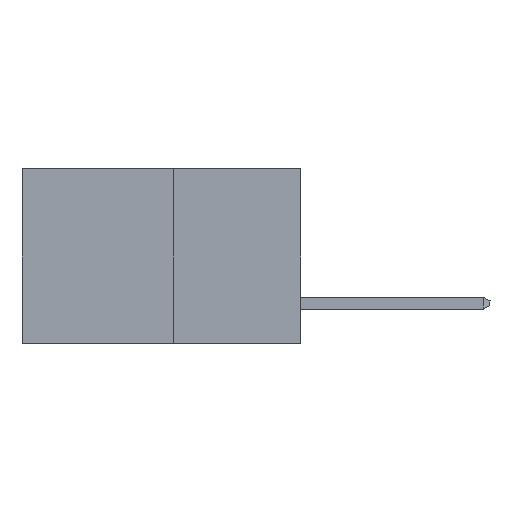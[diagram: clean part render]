
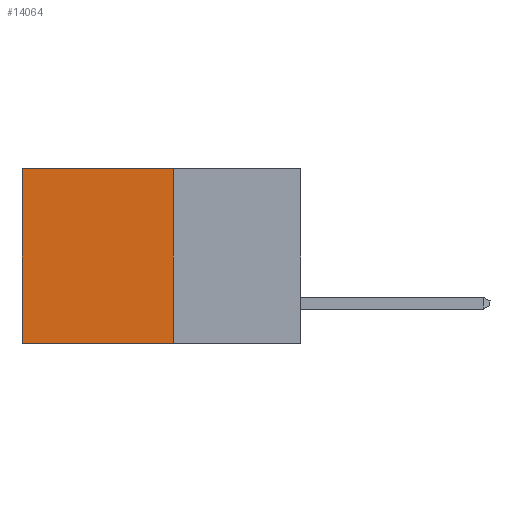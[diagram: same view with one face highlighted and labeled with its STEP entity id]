
A CAD part, left-side view. The second image highlights one B-rep face of the part: STEP entity #14064.
In plain terms, the highlighted planar face has unit normal (-1, 0, 0).
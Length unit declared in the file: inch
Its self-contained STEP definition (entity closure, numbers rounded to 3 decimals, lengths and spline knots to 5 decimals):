
#229 = ORIENTED_EDGE ( 'NONE', *, *, #17463, .F. ) ;
#1659 = VECTOR ( 'NONE', #18160, 39.37008 ) ;
#1755 = DIRECTION ( 'NONE',  ( 0., 1., 0. ) ) ;
#2452 = LINE ( 'NONE', #6009, #1659 ) ;
#3573 = DIRECTION ( 'NONE',  ( 1., 0., 0. ) ) ;
#4290 = LINE ( 'NONE', #23374, #28162 ) ;
#5019 = LINE ( 'NONE', #24667, #23344 ) ;
#5097 = CARTESIAN_POINT ( 'NONE',  ( 0.277, 0.59, 0. ) ) ;
#6009 = CARTESIAN_POINT ( 'NONE',  ( 0.277, 0.27, -0.37 ) ) ;
#6971 = VECTOR ( 'NONE', #15174, 39.37008 ) ;
#7074 = EDGE_CURVE ( 'NONE', #9662, #13632, #20479, .T. ) ;
#8551 = EDGE_LOOP ( 'NONE', ( #28780, #25128, #229, #24511 ) ) ;
#9662 = VERTEX_POINT ( 'NONE', #5097 ) ;
#10799 = PLANE ( 'NONE',  #11037 ) ;
#11037 = AXIS2_PLACEMENT_3D ( 'NONE', #24956, #3573, #20393 ) ;
#11593 = VERTEX_POINT ( 'NONE', #11959 ) ;
#11959 = CARTESIAN_POINT ( 'NONE',  ( 0.277, 0.27, -0.37 ) ) ;
#13632 = VERTEX_POINT ( 'NONE', #13895 ) ;
#13895 = CARTESIAN_POINT ( 'NONE',  ( 0.277, 0.59, -0.37 ) ) ;
#14064 = ADVANCED_FACE ( 'NONE', ( #22107 ), #10799, .F. ) ;
#15174 = DIRECTION ( 'NONE',  ( 0., 0., -1. ) ) ;
#17062 = EDGE_CURVE ( 'NONE', #23329, #9662, #4290, .T. ) ;
#17463 = EDGE_CURVE ( 'NONE', #23329, #11593, #5019, .T. ) ;
#18160 = DIRECTION ( 'NONE',  ( 0., 1., 0. ) ) ;
#20393 = DIRECTION ( 'NONE',  ( 0., 0., -1. ) ) ;
#20479 = LINE ( 'NONE', #24603, #6971 ) ;
#22107 = FACE_OUTER_BOUND ( 'NONE', #8551, .T. ) ;
#22429 = DIRECTION ( 'NONE',  ( 0., 0., -1. ) ) ;
#23329 = VERTEX_POINT ( 'NONE', #24039 ) ;
#23344 = VECTOR ( 'NONE', #22429, 39.37008 ) ;
#23374 = CARTESIAN_POINT ( 'NONE',  ( 0.277, 0.27, 0. ) ) ;
#24039 = CARTESIAN_POINT ( 'NONE',  ( 0.277, 0.27, 0. ) ) ;
#24511 = ORIENTED_EDGE ( 'NONE', *, *, #17062, .T. ) ;
#24603 = CARTESIAN_POINT ( 'NONE',  ( 0.277, 0.59, -0.37 ) ) ;
#24667 = CARTESIAN_POINT ( 'NONE',  ( 0.277, 0.27, -0.37 ) ) ;
#24956 = CARTESIAN_POINT ( 'NONE',  ( 0.277, 0.27, -0.37 ) ) ;
#25128 = ORIENTED_EDGE ( 'NONE', *, *, #28934, .F. ) ;
#28162 = VECTOR ( 'NONE', #1755, 39.37008 ) ;
#28780 = ORIENTED_EDGE ( 'NONE', *, *, #7074, .T. ) ;
#28934 = EDGE_CURVE ( 'NONE', #11593, #13632, #2452, .T. ) ;
